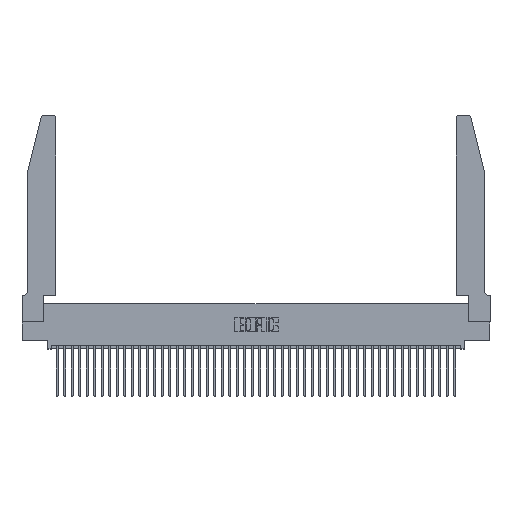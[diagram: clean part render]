
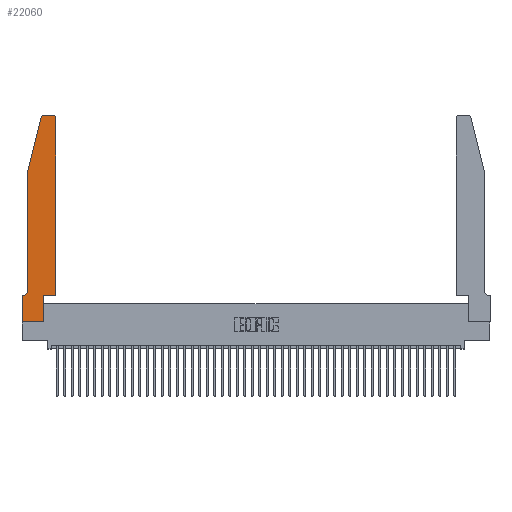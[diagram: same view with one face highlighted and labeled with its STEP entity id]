
A CAD part, top view. The second image highlights one B-rep face of the part: STEP entity #22060.
In plain terms, the highlighted planar face has unit normal (0, 0, 1).
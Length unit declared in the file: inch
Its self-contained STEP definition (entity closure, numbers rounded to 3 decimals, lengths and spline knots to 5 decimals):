
#1201 = ORIENTED_EDGE ( 'NONE', *, *, #3340, .T. ) ;
#1696 = DIRECTION ( 'NONE',  ( -1., 0., 0. ) ) ;
#2669 = VERTEX_POINT ( 'NONE', #29691 ) ;
#2724 = DIRECTION ( 'NONE',  ( -0.239, -0.971, 0. ) ) ;
#3293 = CIRCLE ( 'NONE', #24855, 0.07 ) ;
#3340 = EDGE_CURVE ( 'NONE', #7954, #33325, #14972, .T. ) ;
#4435 = ORIENTED_EDGE ( 'NONE', *, *, #41729, .T. ) ;
#4495 = EDGE_CURVE ( 'NONE', #24669, #8306, #28127, .T. ) ;
#5285 = VECTOR ( 'NONE', #36512, 39.37008 ) ;
#5522 = DIRECTION ( 'NONE',  ( 1., 0., 0. ) ) ;
#6567 = CARTESIAN_POINT ( 'NONE',  ( 0.2865, 0.35, 0.37 ) ) ;
#7316 = ORIENTED_EDGE ( 'NONE', *, *, #33863, .T. ) ;
#7780 = DIRECTION ( 'NONE',  ( 0., 0., -1. ) ) ;
#7954 = VERTEX_POINT ( 'NONE', #20639 ) ;
#8306 = VERTEX_POINT ( 'NONE', #18586 ) ;
#8319 = CARTESIAN_POINT ( 'NONE',  ( 0.4505, 0.35, 0.37 ) ) ;
#9151 = CARTESIAN_POINT ( 'NONE',  ( 0.0055, 0.35, 0.37 ) ) ;
#9451 = CARTESIAN_POINT ( 'NONE',  ( 0.0755, 2., 0.37 ) ) ;
#10273 = LINE ( 'NONE', #8319, #5285 ) ;
#10561 = LINE ( 'NONE', #9451, #27139 ) ;
#11537 = ORIENTED_EDGE ( 'NONE', *, *, #32706, .T. ) ;
#12016 = DIRECTION ( 'NONE',  ( 0., 0., 1. ) ) ;
#12364 = VERTEX_POINT ( 'NONE', #40403 ) ;
#12680 = EDGE_CURVE ( 'NONE', #8306, #34120, #10561, .T. ) ;
#12846 = EDGE_CURVE ( 'NONE', #34120, #2669, #22692, .T. ) ;
#12936 = CARTESIAN_POINT ( 'NONE',  ( 0., 0., 0.37 ) ) ;
#13819 = CARTESIAN_POINT ( 'NONE',  ( 0., 0., 0.37 ) ) ;
#14826 = DIRECTION ( 'NONE',  ( 0., 1., 0. ) ) ;
#14953 = VERTEX_POINT ( 'NONE', #21213 ) ;
#14972 = LINE ( 'NONE', #12936, #21055 ) ;
#15265 = EDGE_CURVE ( 'NONE', #25259, #21793, #25677, .T. ) ;
#17489 = ORIENTED_EDGE ( 'NONE', *, *, #4495, .T. ) ;
#17926 = DIRECTION ( 'NONE',  ( -1., 0., 0. ) ) ;
#18485 = EDGE_CURVE ( 'NONE', #19989, #25259, #28205, .T. ) ;
#18586 = CARTESIAN_POINT ( 'NONE',  ( 0.25487, 2.72718, 0.37 ) ) ;
#18913 = CIRCLE ( 'NONE', #42088, 0.03 ) ;
#19126 = PLANE ( 'NONE',  #37186 ) ;
#19611 = CARTESIAN_POINT ( 'NONE',  ( 0.4205, 2.72, 0.37 ) ) ;
#19989 = VERTEX_POINT ( 'NONE', #37813 ) ;
#20639 = CARTESIAN_POINT ( 'NONE',  ( 0., 0.35, 0.37 ) ) ;
#21055 = VECTOR ( 'NONE', #37869, 39.37008 ) ;
#21213 = CARTESIAN_POINT ( 'NONE',  ( 0.4205, 2.75, 0.37 ) ) ;
#21604 = VERTEX_POINT ( 'NONE', #9151 ) ;
#21793 = VERTEX_POINT ( 'NONE', #28413 ) ;
#22060 = ADVANCED_FACE ( 'NONE', ( #23292 ), #19126, .T. ) ;
#22379 = CARTESIAN_POINT ( 'NONE',  ( 0., 0.35, 0.37 ) ) ;
#22692 = LINE ( 'NONE', #42066, #25444 ) ;
#22735 = CARTESIAN_POINT ( 'NONE',  ( 0.2605, 2.75, 0.37 ) ) ;
#23241 = ORIENTED_EDGE ( 'NONE', *, *, #37828, .T. ) ;
#23256 = LINE ( 'NONE', #22735, #35333 ) ;
#23292 = FACE_OUTER_BOUND ( 'NONE', #35835, .T. ) ;
#23760 = CARTESIAN_POINT ( 'NONE',  ( 0.284, 2.72, 0.37 ) ) ;
#23805 = VECTOR ( 'NONE', #41714, 39.37008 ) ;
#24373 = DIRECTION ( 'NONE',  ( 0., 0., 1. ) ) ;
#24669 = VERTEX_POINT ( 'NONE', #42061 ) ;
#24855 = AXIS2_PLACEMENT_3D ( 'NONE', #28608, #7780, #32433 ) ;
#24886 = EDGE_CURVE ( 'NONE', #21793, #12364, #10273, .T. ) ;
#25259 = VERTEX_POINT ( 'NONE', #6567 ) ;
#25444 = VECTOR ( 'NONE', #39905, 39.37008 ) ;
#25677 = LINE ( 'NONE', #34133, #43871 ) ;
#27139 = VECTOR ( 'NONE', #2724, 39.37008 ) ;
#27250 = ORIENTED_EDGE ( 'NONE', *, *, #18485, .T. ) ;
#27501 = CARTESIAN_POINT ( 'NONE',  ( 0.0755, 2., 0.37 ) ) ;
#28127 = CIRCLE ( 'NONE', #29028, 0.03 ) ;
#28205 = LINE ( 'NONE', #36403, #39730 ) ;
#28413 = CARTESIAN_POINT ( 'NONE',  ( 0.4505, 0.35, 0.37 ) ) ;
#28608 = CARTESIAN_POINT ( 'NONE',  ( 0.0055, 0.42, 0.37 ) ) ;
#29028 = AXIS2_PLACEMENT_3D ( 'NONE', #23760, #24373, #34517 ) ;
#29414 = EDGE_CURVE ( 'NONE', #33325, #19989, #36467, .T. ) ;
#29691 = CARTESIAN_POINT ( 'NONE',  ( 0.0755, 0.42, 0.37 ) ) ;
#31645 = CARTESIAN_POINT ( 'NONE',  ( 0.0755, 0.35, 0.37 ) ) ;
#32433 = DIRECTION ( 'NONE',  ( -1., 0., 0. ) ) ;
#32540 = ORIENTED_EDGE ( 'NONE', *, *, #24886, .T. ) ;
#32706 = EDGE_CURVE ( 'NONE', #12364, #14953, #18913, .T. ) ;
#33325 = VERTEX_POINT ( 'NONE', #44482 ) ;
#33506 = VECTOR ( 'NONE', #17926, 39.37008 ) ;
#33863 = EDGE_CURVE ( 'NONE', #14953, #24669, #23256, .T. ) ;
#34120 = VERTEX_POINT ( 'NONE', #27501 ) ;
#34133 = CARTESIAN_POINT ( 'NONE',  ( 0.4505, 0.35, 0.37 ) ) ;
#34517 = DIRECTION ( 'NONE',  ( 1., 0., 0. ) ) ;
#34775 = ORIENTED_EDGE ( 'NONE', *, *, #29414, .T. ) ;
#35333 = VECTOR ( 'NONE', #1696, 39.37008 ) ;
#35835 = EDGE_LOOP ( 'NONE', ( #7316, #17489, #44424, #42360, #23241, #4435, #1201, #34775, #27250, #36308, #32540, #11537 ) ) ;
#36308 = ORIENTED_EDGE ( 'NONE', *, *, #15265, .T. ) ;
#36403 = CARTESIAN_POINT ( 'NONE',  ( 0.2865, 0.35, 0.37 ) ) ;
#36467 = LINE ( 'NONE', #13819, #23805 ) ;
#36512 = DIRECTION ( 'NONE',  ( 0., 1., 0. ) ) ;
#36524 = DIRECTION ( 'NONE',  ( 1., 0., 0. ) ) ;
#37186 = AXIS2_PLACEMENT_3D ( 'NONE', #22379, #12016, #36524 ) ;
#37813 = CARTESIAN_POINT ( 'NONE',  ( 0.2865, 0., 0.37 ) ) ;
#37828 = EDGE_CURVE ( 'NONE', #2669, #21604, #3293, .T. ) ;
#37869 = DIRECTION ( 'NONE',  ( 0., -1., 0. ) ) ;
#39730 = VECTOR ( 'NONE', #14826, 39.37008 ) ;
#39905 = DIRECTION ( 'NONE',  ( 0., -1., 0. ) ) ;
#40403 = CARTESIAN_POINT ( 'NONE',  ( 0.4505, 2.72, 0.37 ) ) ;
#40751 = DIRECTION ( 'NONE',  ( 1., 0., 0. ) ) ;
#41714 = DIRECTION ( 'NONE',  ( 1., 0., 0. ) ) ;
#41729 = EDGE_CURVE ( 'NONE', #21604, #7954, #42844, .T. ) ;
#42061 = CARTESIAN_POINT ( 'NONE',  ( 0.284, 2.75, 0.37 ) ) ;
#42066 = CARTESIAN_POINT ( 'NONE',  ( 0.0755, 2., 0.37 ) ) ;
#42088 = AXIS2_PLACEMENT_3D ( 'NONE', #19611, #44245, #5522 ) ;
#42360 = ORIENTED_EDGE ( 'NONE', *, *, #12846, .T. ) ;
#42844 = LINE ( 'NONE', #31645, #33506 ) ;
#43871 = VECTOR ( 'NONE', #40751, 39.37008 ) ;
#44245 = DIRECTION ( 'NONE',  ( 0., 0., 1. ) ) ;
#44424 = ORIENTED_EDGE ( 'NONE', *, *, #12680, .T. ) ;
#44482 = CARTESIAN_POINT ( 'NONE',  ( 0., 0., 0.37 ) ) ;
